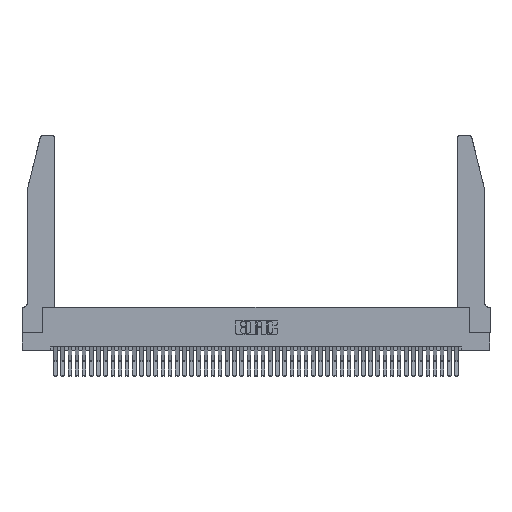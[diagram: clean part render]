
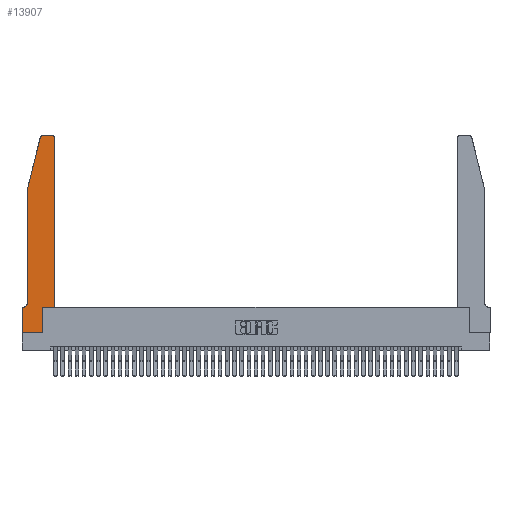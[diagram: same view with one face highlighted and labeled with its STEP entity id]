
A CAD part, top view. The second image highlights one B-rep face of the part: STEP entity #13907.
In plain terms, the highlighted planar face has unit normal (0, 0, 1).
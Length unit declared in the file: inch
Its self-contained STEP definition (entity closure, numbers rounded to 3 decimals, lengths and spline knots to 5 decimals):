
#563 = LINE ( 'NONE', #31853, #19143 ) ;
#1840 = CARTESIAN_POINT ( 'NONE',  ( 0.0055, 0.35, 0.37 ) ) ;
#2225 = VECTOR ( 'NONE', #34381, 39.37008 ) ;
#2443 = CARTESIAN_POINT ( 'NONE',  ( 0.0055, 0.42, 0.37 ) ) ;
#2552 = CARTESIAN_POINT ( 'NONE',  ( 0.0755, 0.42, 0.37 ) ) ;
#2647 = CARTESIAN_POINT ( 'NONE',  ( 0.0755, 0.35, 0.37 ) ) ;
#4089 = EDGE_CURVE ( 'NONE', #18949, #4645, #46932, .T. ) ;
#4526 = ORIENTED_EDGE ( 'NONE', *, *, #24300, .T. ) ;
#4645 = VERTEX_POINT ( 'NONE', #27946 ) ;
#5711 = EDGE_CURVE ( 'NONE', #32157, #24041, #6350, .T. ) ;
#6236 = DIRECTION ( 'NONE',  ( -1., 0., 0. ) ) ;
#6350 = LINE ( 'NONE', #34226, #35643 ) ;
#7051 = CARTESIAN_POINT ( 'NONE',  ( 0.4205, 2.72, 0.37 ) ) ;
#7573 = LINE ( 'NONE', #24917, #35690 ) ;
#7701 = CIRCLE ( 'NONE', #46808, 0.07 ) ;
#8327 = EDGE_LOOP ( 'NONE', ( #38702, #4526, #23194, #26044, #47015, #30526, #29285, #21792, #10272, #43115, #21921, #46136 ) ) ;
#8387 = DIRECTION ( 'NONE',  ( 0., -1., 0. ) ) ;
#8741 = CARTESIAN_POINT ( 'NONE',  ( 0.4505, 0.35, 0.37 ) ) ;
#9105 = CARTESIAN_POINT ( 'NONE',  ( 0.284, 2.72, 0.37 ) ) ;
#10170 = DIRECTION ( 'NONE',  ( -1., 0., 0. ) ) ;
#10272 = ORIENTED_EDGE ( 'NONE', *, *, #30423, .T. ) ;
#10684 = VECTOR ( 'NONE', #40392, 39.37008 ) ;
#10779 = DIRECTION ( 'NONE',  ( 1., 0., 0. ) ) ;
#11434 = EDGE_CURVE ( 'NONE', #39281, #40141, #563, .T. ) ;
#11826 = LINE ( 'NONE', #36738, #10684 ) ;
#12364 = CARTESIAN_POINT ( 'NONE',  ( 0.4505, 2.72, 0.37 ) ) ;
#12583 = PLANE ( 'NONE',  #32312 ) ;
#12798 = DIRECTION ( 'NONE',  ( 1., 0., 0. ) ) ;
#13722 = VERTEX_POINT ( 'NONE', #37253 ) ;
#13786 = DIRECTION ( 'NONE',  ( -0.239, -0.971, 0. ) ) ;
#13907 = ADVANCED_FACE ( 'NONE', ( #37371 ), #12583, .T. ) ;
#14756 = AXIS2_PLACEMENT_3D ( 'NONE', #9105, #34738, #12798 ) ;
#15973 = DIRECTION ( 'NONE',  ( 1., 0., 0. ) ) ;
#16051 = CARTESIAN_POINT ( 'NONE',  ( 0.25487, 2.72718, 0.37 ) ) ;
#16778 = AXIS2_PLACEMENT_3D ( 'NONE', #7051, #32727, #10779 ) ;
#17109 = DIRECTION ( 'NONE',  ( 0., 1., 0. ) ) ;
#17251 = LINE ( 'NONE', #28401, #45227 ) ;
#17256 = CARTESIAN_POINT ( 'NONE',  ( 0.4505, 0.35, 0.37 ) ) ;
#17675 = DIRECTION ( 'NONE',  ( -1., 0., 0. ) ) ;
#18804 = EDGE_CURVE ( 'NONE', #13722, #39281, #39056, .T. ) ;
#18949 = VERTEX_POINT ( 'NONE', #1840 ) ;
#19126 = CIRCLE ( 'NONE', #14756, 0.03 ) ;
#19143 = VECTOR ( 'NONE', #17109, 39.37008 ) ;
#19457 = CARTESIAN_POINT ( 'NONE',  ( 0.284, 2.75, 0.37 ) ) ;
#19715 = EDGE_CURVE ( 'NONE', #40141, #32027, #41225, .T. ) ;
#19970 = DIRECTION ( 'NONE',  ( 1., 0., 0. ) ) ;
#21253 = DIRECTION ( 'NONE',  ( 0., 1., 0. ) ) ;
#21608 = VERTEX_POINT ( 'NONE', #19457 ) ;
#21661 = VERTEX_POINT ( 'NONE', #16051 ) ;
#21792 = ORIENTED_EDGE ( 'NONE', *, *, #5711, .T. ) ;
#21921 = ORIENTED_EDGE ( 'NONE', *, *, #11434, .T. ) ;
#23194 = ORIENTED_EDGE ( 'NONE', *, *, #42208, .T. ) ;
#24041 = VERTEX_POINT ( 'NONE', #29667 ) ;
#24300 = EDGE_CURVE ( 'NONE', #21608, #21661, #19126, .T. ) ;
#24917 = CARTESIAN_POINT ( 'NONE',  ( 0.2605, 2.75, 0.37 ) ) ;
#25441 = VECTOR ( 'NONE', #8387, 39.37008 ) ;
#26044 = ORIENTED_EDGE ( 'NONE', *, *, #26472, .T. ) ;
#26472 = EDGE_CURVE ( 'NONE', #28468, #32911, #11826, .T. ) ;
#26698 = CARTESIAN_POINT ( 'NONE',  ( 0., 0., 0.37 ) ) ;
#27946 = CARTESIAN_POINT ( 'NONE',  ( 0., 0.35, 0.37 ) ) ;
#28286 = DIRECTION ( 'NONE',  ( 0., 0., -1. ) ) ;
#28401 = CARTESIAN_POINT ( 'NONE',  ( 0.0755, 2., 0.37 ) ) ;
#28468 = VERTEX_POINT ( 'NONE', #43277 ) ;
#28780 = EDGE_CURVE ( 'NONE', #4645, #32157, #35141, .T. ) ;
#29285 = ORIENTED_EDGE ( 'NONE', *, *, #28780, .T. ) ;
#29667 = CARTESIAN_POINT ( 'NONE',  ( 0.2865, 0., 0.37 ) ) ;
#30423 = EDGE_CURVE ( 'NONE', #24041, #13722, #47508, .T. ) ;
#30526 = ORIENTED_EDGE ( 'NONE', *, *, #4089, .T. ) ;
#31618 = CARTESIAN_POINT ( 'NONE',  ( 0., 0., 0.37 ) ) ;
#31853 = CARTESIAN_POINT ( 'NONE',  ( 0.4505, 0.35, 0.37 ) ) ;
#32027 = VERTEX_POINT ( 'NONE', #38176 ) ;
#32157 = VERTEX_POINT ( 'NONE', #31618 ) ;
#32174 = EDGE_CURVE ( 'NONE', #32911, #18949, #7701, .T. ) ;
#32312 = AXIS2_PLACEMENT_3D ( 'NONE', #38185, #41814, #19970 ) ;
#32727 = DIRECTION ( 'NONE',  ( 0., 0., 1. ) ) ;
#32911 = VERTEX_POINT ( 'NONE', #2552 ) ;
#34208 = EDGE_CURVE ( 'NONE', #32027, #21608, #7573, .T. ) ;
#34226 = CARTESIAN_POINT ( 'NONE',  ( 0., 0., 0.37 ) ) ;
#34381 = DIRECTION ( 'NONE',  ( 1., 0., 0. ) ) ;
#34407 = VECTOR ( 'NONE', #21253, 39.37008 ) ;
#34738 = DIRECTION ( 'NONE',  ( 0., 0., 1. ) ) ;
#35141 = LINE ( 'NONE', #26698, #25441 ) ;
#35643 = VECTOR ( 'NONE', #15973, 39.37008 ) ;
#35690 = VECTOR ( 'NONE', #17675, 39.37008 ) ;
#36138 = VECTOR ( 'NONE', #10170, 39.37008 ) ;
#36738 = CARTESIAN_POINT ( 'NONE',  ( 0.0755, 2., 0.37 ) ) ;
#37253 = CARTESIAN_POINT ( 'NONE',  ( 0.2865, 0.35, 0.37 ) ) ;
#37371 = FACE_OUTER_BOUND ( 'NONE', #8327, .T. ) ;
#38176 = CARTESIAN_POINT ( 'NONE',  ( 0.4205, 2.75, 0.37 ) ) ;
#38185 = CARTESIAN_POINT ( 'NONE',  ( 0., 0.35, 0.37 ) ) ;
#38702 = ORIENTED_EDGE ( 'NONE', *, *, #34208, .T. ) ;
#39056 = LINE ( 'NONE', #8741, #2225 ) ;
#39281 = VERTEX_POINT ( 'NONE', #17256 ) ;
#40141 = VERTEX_POINT ( 'NONE', #12364 ) ;
#40392 = DIRECTION ( 'NONE',  ( 0., -1., 0. ) ) ;
#41225 = CIRCLE ( 'NONE', #16778, 0.03 ) ;
#41814 = DIRECTION ( 'NONE',  ( 0., 0., 1. ) ) ;
#42208 = EDGE_CURVE ( 'NONE', #21661, #28468, #17251, .T. ) ;
#43115 = ORIENTED_EDGE ( 'NONE', *, *, #18804, .T. ) ;
#43277 = CARTESIAN_POINT ( 'NONE',  ( 0.0755, 2., 0.37 ) ) ;
#45227 = VECTOR ( 'NONE', #13786, 39.37008 ) ;
#46136 = ORIENTED_EDGE ( 'NONE', *, *, #19715, .T. ) ;
#46710 = CARTESIAN_POINT ( 'NONE',  ( 0.2865, 0.35, 0.37 ) ) ;
#46808 = AXIS2_PLACEMENT_3D ( 'NONE', #2443, #28286, #6236 ) ;
#46932 = LINE ( 'NONE', #2647, #36138 ) ;
#47015 = ORIENTED_EDGE ( 'NONE', *, *, #32174, .T. ) ;
#47508 = LINE ( 'NONE', #46710, #34407 ) ;
